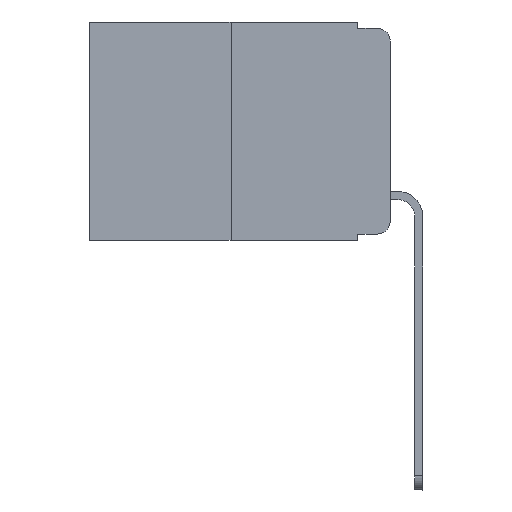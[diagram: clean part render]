
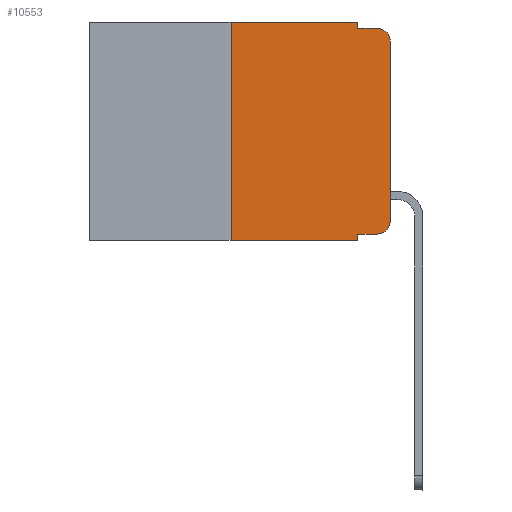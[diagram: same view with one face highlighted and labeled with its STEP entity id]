
A CAD part, left-side view. The second image highlights one B-rep face of the part: STEP entity #10553.
In plain terms, the highlighted planar face has unit normal (-1, 0, 0).
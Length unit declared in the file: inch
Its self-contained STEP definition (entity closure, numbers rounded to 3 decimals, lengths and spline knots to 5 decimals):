
#162 = DIRECTION ( 'NONE',  ( 0., 0., -1. ) ) ;
#198 = DIRECTION ( 'NONE',  ( 0., 0., 1. ) ) ;
#359 = DIRECTION ( 'NONE',  ( -1., 0., 0. ) ) ;
#566 = DIRECTION ( 'NONE',  ( 0., 0., -1. ) ) ;
#736 = VERTEX_POINT ( 'NONE', #9634 ) ;
#973 = VERTEX_POINT ( 'NONE', #7574 ) ;
#1142 = CARTESIAN_POINT ( 'NONE',  ( 0., 0.473, 0. ) ) ;
#1292 = CARTESIAN_POINT ( 'NONE',  ( 0., 0.051, -0.01 ) ) ;
#2229 = CARTESIAN_POINT ( 'NONE',  ( 0., 0., -0.03 ) ) ;
#2808 = VECTOR ( 'NONE', #198, 39.37008 ) ;
#2830 = CIRCLE ( 'NONE', #4437, 0.02 ) ;
#2953 = ORIENTED_EDGE ( 'NONE', *, *, #10167, .T. ) ;
#3558 = EDGE_CURVE ( 'NONE', #18150, #4981, #4779, .T. ) ;
#4280 = LINE ( 'NONE', #10117, #7853 ) ;
#4317 = ORIENTED_EDGE ( 'NONE', *, *, #8650, .F. ) ;
#4437 = AXIS2_PLACEMENT_3D ( 'NONE', #10715, #12070, #14823 ) ;
#4776 = CIRCLE ( 'NONE', #15655, 0.02 ) ;
#4779 = LINE ( 'NONE', #17919, #2808 ) ;
#4918 = VERTEX_POINT ( 'NONE', #10823 ) ;
#4981 = VERTEX_POINT ( 'NONE', #2229 ) ;
#5141 = ORIENTED_EDGE ( 'NONE', *, *, #5337, .F. ) ;
#5337 = EDGE_CURVE ( 'NONE', #736, #4918, #18084, .T. ) ;
#5586 = CARTESIAN_POINT ( 'NONE',  ( 0., 0.473, 0. ) ) ;
#5925 = ORIENTED_EDGE ( 'NONE', *, *, #10177, .T. ) ;
#7076 = DIRECTION ( 'NONE',  ( 1., 0., 0. ) ) ;
#7290 = EDGE_CURVE ( 'NONE', #8444, #736, #8512, .T. ) ;
#7574 = CARTESIAN_POINT ( 'NONE',  ( 0., 0.02, -0.333 ) ) ;
#7724 = CARTESIAN_POINT ( 'NONE',  ( 0., 0.051, -0.333 ) ) ;
#7733 = ORIENTED_EDGE ( 'NONE', *, *, #8293, .F. ) ;
#7810 = VECTOR ( 'NONE', #8173, 39.37008 ) ;
#7834 = VECTOR ( 'NONE', #19115, 39.37008 ) ;
#7853 = VECTOR ( 'NONE', #17626, 39.37008 ) ;
#7886 = LINE ( 'NONE', #13823, #7810 ) ;
#8173 = DIRECTION ( 'NONE',  ( 0., 0., -1. ) ) ;
#8293 = EDGE_CURVE ( 'NONE', #9988, #8444, #16105, .T. ) ;
#8399 = CARTESIAN_POINT ( 'NONE',  ( 0., 0.02, -0.01 ) ) ;
#8444 = VERTEX_POINT ( 'NONE', #9061 ) ;
#8512 = LINE ( 'NONE', #5586, #13379 ) ;
#8650 = EDGE_CURVE ( 'NONE', #17094, #17042, #7886, .T. ) ;
#9061 = CARTESIAN_POINT ( 'NONE',  ( 0., 0.25, 0. ) ) ;
#9634 = CARTESIAN_POINT ( 'NONE',  ( 0., 0.051, 0. ) ) ;
#9730 = ORIENTED_EDGE ( 'NONE', *, *, #12550, .F. ) ;
#9848 = EDGE_CURVE ( 'NONE', #973, #18150, #2830, .T. ) ;
#9988 = VERTEX_POINT ( 'NONE', #14007 ) ;
#10117 = CARTESIAN_POINT ( 'NONE',  ( 0., 0.473, -0.343 ) ) ;
#10167 = EDGE_CURVE ( 'NONE', #17094, #973, #18888, .T. ) ;
#10177 = EDGE_CURVE ( 'NONE', #9988, #17042, #4280, .T. ) ;
#10553 = ADVANCED_FACE ( 'NONE', ( #14479 ), #12906, .F. ) ;
#10682 = EDGE_LOOP ( 'NONE', ( #12375, #16089, #9730, #5141, #18639, #7733, #5925, #4317, #2953, #14482 ) ) ;
#10715 = CARTESIAN_POINT ( 'NONE',  ( 0., 0.02, -0.313 ) ) ;
#10823 = CARTESIAN_POINT ( 'NONE',  ( 0., 0.051, -0.01 ) ) ;
#11504 = DIRECTION ( 'NONE',  ( 0., -1., 0. ) ) ;
#11527 = VECTOR ( 'NONE', #11562, 39.37008 ) ;
#11562 = DIRECTION ( 'NONE',  ( 0., -1., 0. ) ) ;
#11661 = CARTESIAN_POINT ( 'NONE',  ( 0., 0.051, -0.333 ) ) ;
#11963 = EDGE_CURVE ( 'NONE', #4981, #17287, #4776, .T. ) ;
#12070 = DIRECTION ( 'NONE',  ( -1., 0., 0. ) ) ;
#12205 = CARTESIAN_POINT ( 'NONE',  ( 0., 0.051, -0.343 ) ) ;
#12375 = ORIENTED_EDGE ( 'NONE', *, *, #3558, .T. ) ;
#12550 = EDGE_CURVE ( 'NONE', #4918, #17287, #14633, .T. ) ;
#12906 = PLANE ( 'NONE',  #13414 ) ;
#13379 = VECTOR ( 'NONE', #11504, 39.37008 ) ;
#13414 = AXIS2_PLACEMENT_3D ( 'NONE', #1142, #7076, #17400 ) ;
#13823 = CARTESIAN_POINT ( 'NONE',  ( 0., 0.051, 0. ) ) ;
#14007 = CARTESIAN_POINT ( 'NONE',  ( 0., 0.25, -0.343 ) ) ;
#14479 = FACE_OUTER_BOUND ( 'NONE', #10682, .T. ) ;
#14482 = ORIENTED_EDGE ( 'NONE', *, *, #9848, .T. ) ;
#14633 = LINE ( 'NONE', #1292, #7834 ) ;
#14823 = DIRECTION ( 'NONE',  ( 0., 0., -1. ) ) ;
#15331 = VECTOR ( 'NONE', #566, 39.37008 ) ;
#15655 = AXIS2_PLACEMENT_3D ( 'NONE', #17694, #359, #162 ) ;
#16089 = ORIENTED_EDGE ( 'NONE', *, *, #11963, .T. ) ;
#16105 = LINE ( 'NONE', #16192, #16871 ) ;
#16192 = CARTESIAN_POINT ( 'NONE',  ( 0., 0.25, 0. ) ) ;
#16871 = VECTOR ( 'NONE', #18907, 39.37008 ) ;
#17042 = VERTEX_POINT ( 'NONE', #12205 ) ;
#17094 = VERTEX_POINT ( 'NONE', #7724 ) ;
#17287 = VERTEX_POINT ( 'NONE', #8399 ) ;
#17400 = DIRECTION ( 'NONE',  ( 0., 0., -1. ) ) ;
#17626 = DIRECTION ( 'NONE',  ( 0., -1., 0. ) ) ;
#17694 = CARTESIAN_POINT ( 'NONE',  ( 0., 0.02, -0.03 ) ) ;
#17919 = CARTESIAN_POINT ( 'NONE',  ( 0., 0., 0. ) ) ;
#18084 = LINE ( 'NONE', #18285, #15331 ) ;
#18150 = VERTEX_POINT ( 'NONE', #18399 ) ;
#18285 = CARTESIAN_POINT ( 'NONE',  ( 0., 0.051, 0. ) ) ;
#18399 = CARTESIAN_POINT ( 'NONE',  ( 0., 0., -0.313 ) ) ;
#18639 = ORIENTED_EDGE ( 'NONE', *, *, #7290, .F. ) ;
#18888 = LINE ( 'NONE', #11661, #11527 ) ;
#18907 = DIRECTION ( 'NONE',  ( 0., 0., 1. ) ) ;
#19115 = DIRECTION ( 'NONE',  ( 0., -1., 0. ) ) ;
